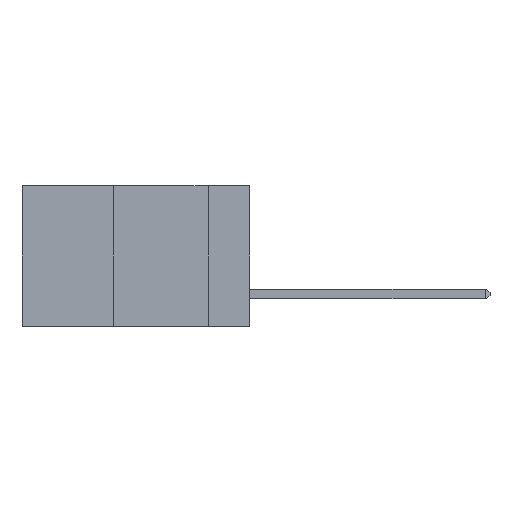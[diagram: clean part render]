
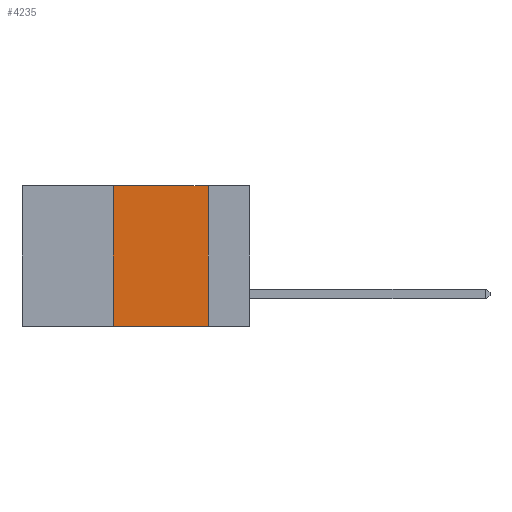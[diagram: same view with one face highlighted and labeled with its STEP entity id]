
A CAD part, left-side view. The second image highlights one B-rep face of the part: STEP entity #4235.
In plain terms, the highlighted planar face has unit normal (-1, 0, 0).
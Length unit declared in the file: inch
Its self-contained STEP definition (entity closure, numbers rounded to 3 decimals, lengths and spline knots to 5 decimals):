
#863 = EDGE_CURVE ( 'NONE', #18537, #5585, #18419, .T. ) ;
#2534 = VECTOR ( 'NONE', #17201, 39.37008 ) ;
#2701 = ORIENTED_EDGE ( 'NONE', *, *, #11544, .F. ) ;
#2713 = ORIENTED_EDGE ( 'NONE', *, *, #6615, .F. ) ;
#2807 = ORIENTED_EDGE ( 'NONE', *, *, #9719, .F. ) ;
#2837 = ORIENTED_EDGE ( 'NONE', *, *, #863, .T. ) ;
#3006 = LINE ( 'NONE', #15671, #2534 ) ;
#3639 = VECTOR ( 'NONE', #16748, 39.37008 ) ;
#4235 = ADVANCED_FACE ( 'NONE', ( #19687 ), #7870, .F. ) ;
#4572 = CARTESIAN_POINT ( 'NONE',  ( 0., 0.11, 0. ) ) ;
#4832 = DIRECTION ( 'NONE',  ( 0., 0., -1. ) ) ;
#5355 = VECTOR ( 'NONE', #16946, 39.37008 ) ;
#5585 = VERTEX_POINT ( 'NONE', #18995 ) ;
#6550 = CARTESIAN_POINT ( 'NONE',  ( 0., 0.36, 0. ) ) ;
#6615 = EDGE_CURVE ( 'NONE', #19301, #18913, #3006, .T. ) ;
#7870 = PLANE ( 'NONE',  #9603 ) ;
#9603 = AXIS2_PLACEMENT_3D ( 'NONE', #12604, #14124, #4832 ) ;
#9719 = EDGE_CURVE ( 'NONE', #18537, #19301, #12613, .T. ) ;
#9793 = CARTESIAN_POINT ( 'NONE',  ( 0., 0.36, -0.37 ) ) ;
#11544 = EDGE_CURVE ( 'NONE', #18913, #5585, #13608, .T. ) ;
#12604 = CARTESIAN_POINT ( 'NONE',  ( 0., 0.6, 0. ) ) ;
#12613 = LINE ( 'NONE', #13641, #3639 ) ;
#13510 = EDGE_LOOP ( 'NONE', ( #2701, #2713, #2807, #2837 ) ) ;
#13608 = LINE ( 'NONE', #4572, #5355 ) ;
#13625 = CARTESIAN_POINT ( 'NONE',  ( 0., 0.11, 0. ) ) ;
#13641 = CARTESIAN_POINT ( 'NONE',  ( 0., 0.36, 0. ) ) ;
#14124 = DIRECTION ( 'NONE',  ( 1., 0., 0. ) ) ;
#14367 = VECTOR ( 'NONE', #14624, 39.37008 ) ;
#14594 = CARTESIAN_POINT ( 'NONE',  ( 0., 0.6, -0.37 ) ) ;
#14624 = DIRECTION ( 'NONE',  ( 0., -1., 0. ) ) ;
#15671 = CARTESIAN_POINT ( 'NONE',  ( 0., 0.6, 0. ) ) ;
#16748 = DIRECTION ( 'NONE',  ( 0., 0., 1. ) ) ;
#16946 = DIRECTION ( 'NONE',  ( 0., 0., -1. ) ) ;
#17201 = DIRECTION ( 'NONE',  ( 0., -1., 0. ) ) ;
#18419 = LINE ( 'NONE', #14594, #14367 ) ;
#18537 = VERTEX_POINT ( 'NONE', #9793 ) ;
#18913 = VERTEX_POINT ( 'NONE', #13625 ) ;
#18995 = CARTESIAN_POINT ( 'NONE',  ( 0., 0.11, -0.37 ) ) ;
#19301 = VERTEX_POINT ( 'NONE', #6550 ) ;
#19687 = FACE_OUTER_BOUND ( 'NONE', #13510, .T. ) ;
